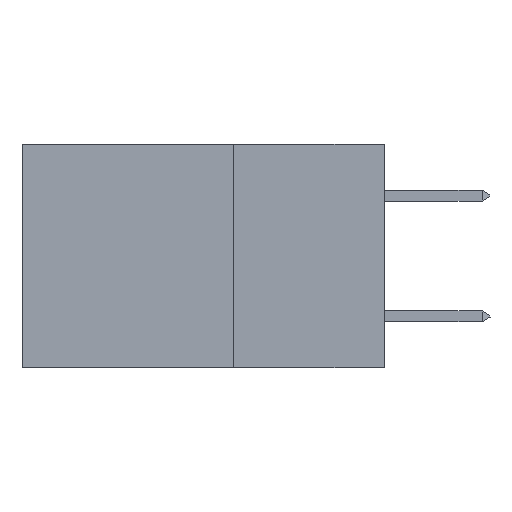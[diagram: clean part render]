
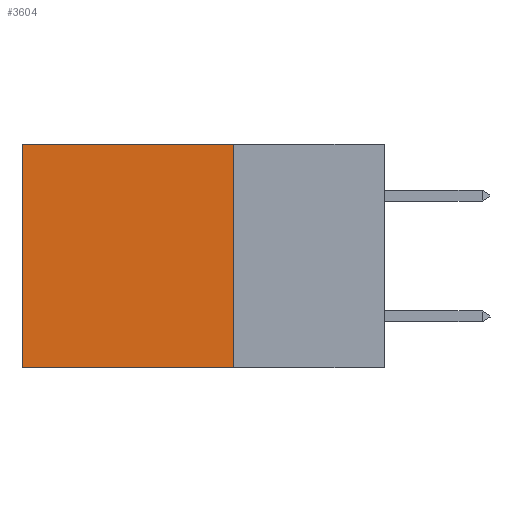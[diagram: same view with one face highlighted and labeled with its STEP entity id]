
A CAD part, left-side view. The second image highlights one B-rep face of the part: STEP entity #3604.
In plain terms, the highlighted planar face has unit normal (-1, 0, 0).
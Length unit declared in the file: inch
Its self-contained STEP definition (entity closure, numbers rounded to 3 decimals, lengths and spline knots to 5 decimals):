
#428 = LINE ( 'NONE', #17269, #20212 ) ;
#734 = FACE_OUTER_BOUND ( 'NONE', #10406, .T. ) ;
#779 = DIRECTION ( 'NONE',  ( 0., 1., 0. ) ) ;
#1433 = VECTOR ( 'NONE', #779, 39.37008 ) ;
#3215 = DIRECTION ( 'NONE',  ( 0., 1., 0. ) ) ;
#3604 = ADVANCED_FACE ( 'NONE', ( #734 ), #3799, .F. ) ;
#3799 = PLANE ( 'NONE',  #5693 ) ;
#5332 = VERTEX_POINT ( 'NONE', #23121 ) ;
#5693 = AXIS2_PLACEMENT_3D ( 'NONE', #11004, #12881, #5914 ) ;
#5914 = DIRECTION ( 'NONE',  ( 0., 0., -1. ) ) ;
#6820 = LINE ( 'NONE', #18727, #1433 ) ;
#7075 = CARTESIAN_POINT ( 'NONE',  ( 0.2875, 0.25, -0.37 ) ) ;
#7429 = LINE ( 'NONE', #7075, #17326 ) ;
#7560 = DIRECTION ( 'NONE',  ( 0., 0., -1. ) ) ;
#8288 = ORIENTED_EDGE ( 'NONE', *, *, #16619, .F. ) ;
#9270 = EDGE_CURVE ( 'NONE', #13489, #15001, #6820, .T. ) ;
#10406 = EDGE_LOOP ( 'NONE', ( #20153, #18655, #8288, #19842 ) ) ;
#10527 = CARTESIAN_POINT ( 'NONE',  ( 0.2875, 0.6, -0.37 ) ) ;
#11004 = CARTESIAN_POINT ( 'NONE',  ( 0.2875, 0.25, 0. ) ) ;
#12881 = DIRECTION ( 'NONE',  ( 1., 0., 0. ) ) ;
#12931 = CARTESIAN_POINT ( 'NONE',  ( 0.2875, 0.6, 0. ) ) ;
#12945 = EDGE_CURVE ( 'NONE', #5332, #21362, #7429, .T. ) ;
#13359 = EDGE_CURVE ( 'NONE', #15001, #21362, #21294, .T. ) ;
#13489 = VERTEX_POINT ( 'NONE', #17109 ) ;
#15001 = VERTEX_POINT ( 'NONE', #23014 ) ;
#16619 = EDGE_CURVE ( 'NONE', #13489, #5332, #428, .T. ) ;
#17109 = CARTESIAN_POINT ( 'NONE',  ( 0.2875, 0.25, 0. ) ) ;
#17269 = CARTESIAN_POINT ( 'NONE',  ( 0.2875, 0.25, 0. ) ) ;
#17326 = VECTOR ( 'NONE', #3215, 39.37008 ) ;
#18655 = ORIENTED_EDGE ( 'NONE', *, *, #12945, .F. ) ;
#18727 = CARTESIAN_POINT ( 'NONE',  ( 0.2875, 0.25, 0. ) ) ;
#19074 = DIRECTION ( 'NONE',  ( 0., 0., -1. ) ) ;
#19842 = ORIENTED_EDGE ( 'NONE', *, *, #9270, .T. ) ;
#20101 = VECTOR ( 'NONE', #7560, 39.37008 ) ;
#20153 = ORIENTED_EDGE ( 'NONE', *, *, #13359, .T. ) ;
#20212 = VECTOR ( 'NONE', #19074, 39.37008 ) ;
#21294 = LINE ( 'NONE', #12931, #20101 ) ;
#21362 = VERTEX_POINT ( 'NONE', #10527 ) ;
#23014 = CARTESIAN_POINT ( 'NONE',  ( 0.2875, 0.6, 0. ) ) ;
#23121 = CARTESIAN_POINT ( 'NONE',  ( 0.2875, 0.25, -0.37 ) ) ;
